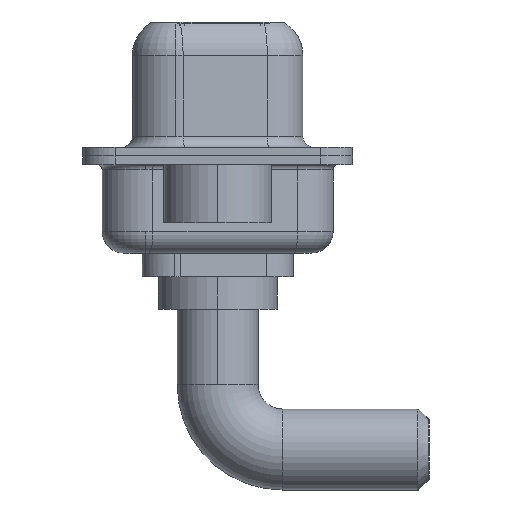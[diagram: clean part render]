
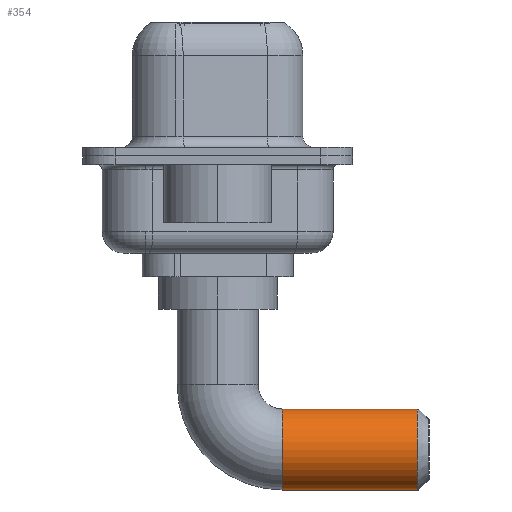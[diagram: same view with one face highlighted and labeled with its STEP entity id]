
A CAD part, left-side view. The second image highlights one B-rep face of the part: STEP entity #354.
In plain terms, the highlighted cylindrical face has radius 1.875 mm (diameter 3.75 mm), a partial arc.
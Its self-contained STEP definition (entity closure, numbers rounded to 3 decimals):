
#280 = EDGE_LOOP ( 'NONE', ( #3927, #5941, #7436, #5090 ) ) ;
#354 = ADVANCED_FACE ( 'NONE', ( #9070 ), #1767, .T. ) ;
#456 = DIRECTION ( 'NONE',  ( 0., -1., 0. ) ) ;
#810 = VECTOR ( 'NONE', #886, 1000. ) ;
#886 = DIRECTION ( 'NONE',  ( 0., -1., 0. ) ) ;
#904 = DIRECTION ( 'NONE',  ( -1., 0., 0. ) ) ;
#1174 = VERTEX_POINT ( 'NONE', #7034 ) ;
#1597 = CARTESIAN_POINT ( 'NONE',  ( 0., -3., -8.375 ) ) ;
#1767 = CYLINDRICAL_SURFACE ( 'NONE', #10618, 1.875 ) ;
#3563 = CARTESIAN_POINT ( 'NONE',  ( 0., -9.25, -6.5 ) ) ;
#3793 = DIRECTION ( 'NONE',  ( 0., 0., -1. ) ) ;
#3927 = ORIENTED_EDGE ( 'NONE', *, *, #10094, .F. ) ;
#4375 = CARTESIAN_POINT ( 'NONE',  ( 0., -3., -8.375 ) ) ;
#4999 = VERTEX_POINT ( 'NONE', #7538 ) ;
#5090 = ORIENTED_EDGE ( 'NONE', *, *, #9175, .T. ) ;
#5337 = CARTESIAN_POINT ( 'NONE',  ( 0., -9.25, -4.625 ) ) ;
#5366 = DIRECTION ( 'NONE',  ( 0., -1., 0. ) ) ;
#5750 = CARTESIAN_POINT ( 'NONE',  ( 0., -3., -6.5 ) ) ;
#5941 = ORIENTED_EDGE ( 'NONE', *, *, #11601, .T. ) ;
#6028 = AXIS2_PLACEMENT_3D ( 'NONE', #6258, #5366, #904 ) ;
#6258 = CARTESIAN_POINT ( 'NONE',  ( 0., -3., -6.5 ) ) ;
#7034 = CARTESIAN_POINT ( 'NONE',  ( 0., -3., -4.625 ) ) ;
#7436 = ORIENTED_EDGE ( 'NONE', *, *, #9908, .T. ) ;
#7538 = CARTESIAN_POINT ( 'NONE',  ( 0., -9.25, -8.375 ) ) ;
#8486 = VERTEX_POINT ( 'NONE', #4375 ) ;
#9040 = VERTEX_POINT ( 'NONE', #5337 ) ;
#9070 = FACE_OUTER_BOUND ( 'NONE', #280, .T. ) ;
#9175 = EDGE_CURVE ( 'NONE', #4999, #9040, #11357, .T. ) ;
#9346 = CIRCLE ( 'NONE', #6028, 1.875 ) ;
#9862 = LINE ( 'NONE', #1597, #12798 ) ;
#9908 = EDGE_CURVE ( 'NONE', #8486, #4999, #9862, .T. ) ;
#10094 = EDGE_CURVE ( 'NONE', #1174, #9040, #10187, .T. ) ;
#10187 = LINE ( 'NONE', #10393, #810 ) ;
#10393 = CARTESIAN_POINT ( 'NONE',  ( 0., -3., -4.625 ) ) ;
#10618 = AXIS2_PLACEMENT_3D ( 'NONE', #5750, #456, #3793 ) ;
#11357 = CIRCLE ( 'NONE', #12038, 1.875 ) ;
#11601 = EDGE_CURVE ( 'NONE', #1174, #8486, #9346, .T. ) ;
#11952 = DIRECTION ( 'NONE',  ( 0., 1., 0. ) ) ;
#12038 = AXIS2_PLACEMENT_3D ( 'NONE', #3563, #11952, #13021 ) ;
#12158 = DIRECTION ( 'NONE',  ( 0., -1., 0. ) ) ;
#12798 = VECTOR ( 'NONE', #12158, 1000. ) ;
#13021 = DIRECTION ( 'NONE',  ( 0., 0., -1. ) ) ;
